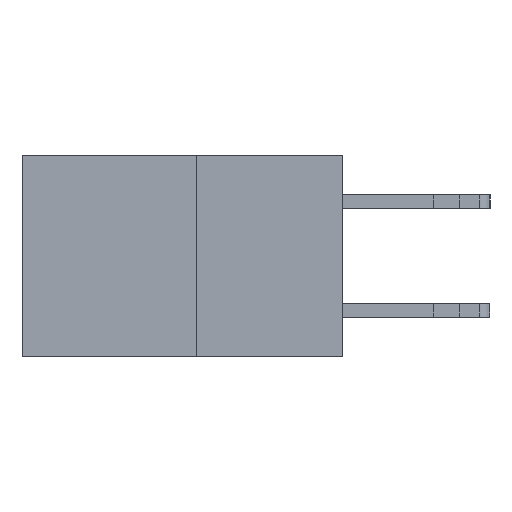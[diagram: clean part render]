
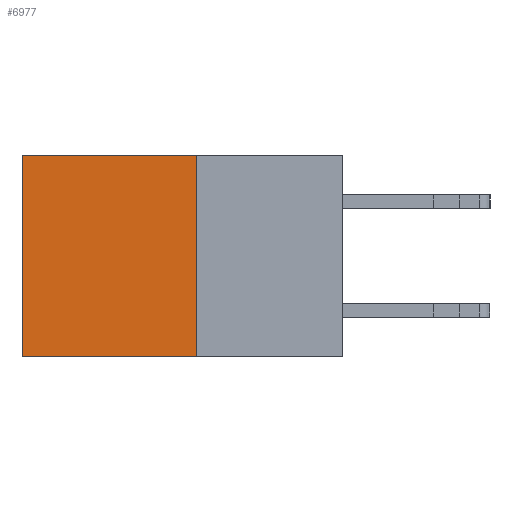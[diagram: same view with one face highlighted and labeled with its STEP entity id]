
A CAD part, left-side view. The second image highlights one B-rep face of the part: STEP entity #6977.
In plain terms, the highlighted planar face has unit normal (-1, 0, 0).
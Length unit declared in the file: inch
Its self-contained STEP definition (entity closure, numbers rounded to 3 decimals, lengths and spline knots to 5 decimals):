
#505 = DIRECTION ( 'NONE',  ( 0., 0., -1. ) ) ;
#564 = DIRECTION ( 'NONE',  ( 0., 1., 0. ) ) ;
#742 = CARTESIAN_POINT ( 'NONE',  ( 0.277, 0.27, 0. ) ) ;
#755 = CARTESIAN_POINT ( 'NONE',  ( 0.277, 0.27, 0. ) ) ;
#799 = VERTEX_POINT ( 'NONE', #10389 ) ;
#2807 = VECTOR ( 'NONE', #15182, 39.37008 ) ;
#2888 = EDGE_CURVE ( 'NONE', #7658, #9406, #10733, .T. ) ;
#3837 = CARTESIAN_POINT ( 'NONE',  ( 0.277, 0.27, -0.37 ) ) ;
#5251 = EDGE_CURVE ( 'NONE', #14645, #799, #9575, .T. ) ;
#5604 = AXIS2_PLACEMENT_3D ( 'NONE', #8247, #5650, #5609 ) ;
#5609 = DIRECTION ( 'NONE',  ( 0., 0., -1. ) ) ;
#5615 = VECTOR ( 'NONE', #505, 39.37008 ) ;
#5650 = DIRECTION ( 'NONE',  ( 1., 0., 0. ) ) ;
#5926 = CARTESIAN_POINT ( 'NONE',  ( 0.277, 0.27, -0.37 ) ) ;
#6858 = PLANE ( 'NONE',  #5604 ) ;
#6977 = ADVANCED_FACE ( 'NONE', ( #12192 ), #6858, .F. ) ;
#7124 = CARTESIAN_POINT ( 'NONE',  ( 0.277, 0.59, -0.37 ) ) ;
#7658 = VERTEX_POINT ( 'NONE', #11145 ) ;
#8247 = CARTESIAN_POINT ( 'NONE',  ( 0.277, 0.27, -0.37 ) ) ;
#9013 = ORIENTED_EDGE ( 'NONE', *, *, #15758, .T. ) ;
#9406 = VERTEX_POINT ( 'NONE', #15478 ) ;
#9575 = LINE ( 'NONE', #755, #18006 ) ;
#10389 = CARTESIAN_POINT ( 'NONE',  ( 0.277, 0.59, 0. ) ) ;
#10733 = LINE ( 'NONE', #5926, #18566 ) ;
#11145 = CARTESIAN_POINT ( 'NONE',  ( 0.277, 0.27, -0.37 ) ) ;
#11564 = LINE ( 'NONE', #3837, #2807 ) ;
#12192 = FACE_OUTER_BOUND ( 'NONE', #12401, .T. ) ;
#12195 = ORIENTED_EDGE ( 'NONE', *, *, #2888, .F. ) ;
#12210 = ORIENTED_EDGE ( 'NONE', *, *, #13694, .F. ) ;
#12401 = EDGE_LOOP ( 'NONE', ( #9013, #12195, #12210, #13724 ) ) ;
#13694 = EDGE_CURVE ( 'NONE', #14645, #7658, #11564, .T. ) ;
#13724 = ORIENTED_EDGE ( 'NONE', *, *, #5251, .T. ) ;
#14645 = VERTEX_POINT ( 'NONE', #742 ) ;
#15182 = DIRECTION ( 'NONE',  ( 0., 0., -1. ) ) ;
#15478 = CARTESIAN_POINT ( 'NONE',  ( 0.277, 0.59, -0.37 ) ) ;
#15758 = EDGE_CURVE ( 'NONE', #799, #9406, #18806, .T. ) ;
#18006 = VECTOR ( 'NONE', #564, 39.37008 ) ;
#18566 = VECTOR ( 'NONE', #18774, 39.37008 ) ;
#18774 = DIRECTION ( 'NONE',  ( 0., 1., 0. ) ) ;
#18806 = LINE ( 'NONE', #7124, #5615 ) ;
